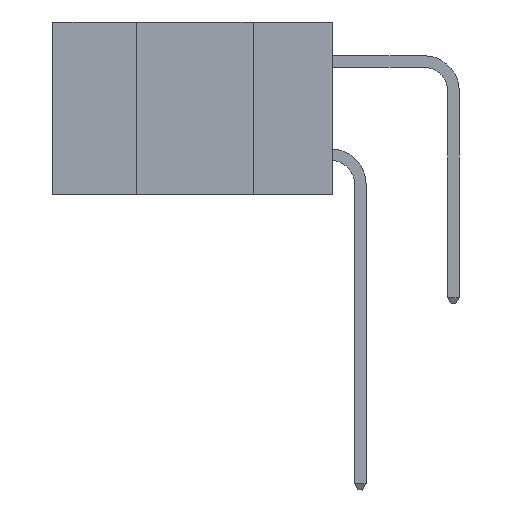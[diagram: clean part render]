
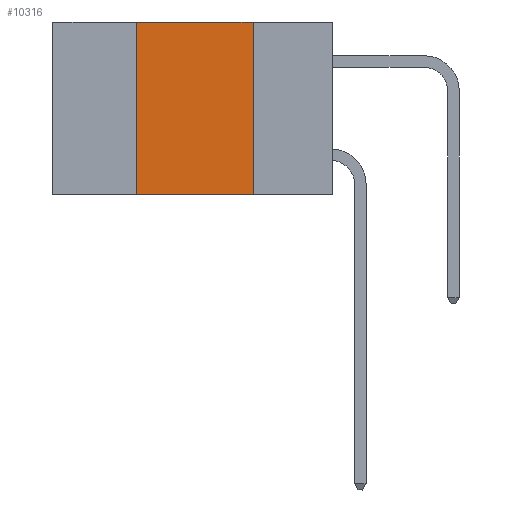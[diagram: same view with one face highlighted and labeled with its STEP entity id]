
A CAD part, left-side view. The second image highlights one B-rep face of the part: STEP entity #10316.
In plain terms, the highlighted planar face has unit normal (-1, 0, 0).
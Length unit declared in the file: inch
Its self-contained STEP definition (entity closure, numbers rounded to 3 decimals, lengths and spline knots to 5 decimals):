
#1430 = CARTESIAN_POINT ( 'NONE',  ( 0., 0.42, 0. ) ) ;
#2302 = LINE ( 'NONE', #6742, #3215 ) ;
#2403 = VECTOR ( 'NONE', #13014, 39.37008 ) ;
#2404 = CARTESIAN_POINT ( 'NONE',  ( 0., 0.6, -0.37 ) ) ;
#2976 = CARTESIAN_POINT ( 'NONE',  ( 0., 0.17, 0. ) ) ;
#3215 = VECTOR ( 'NONE', #18125, 39.37008 ) ;
#3282 = DIRECTION ( 'NONE',  ( 0., 0., 1. ) ) ;
#4327 = LINE ( 'NONE', #2404, #15192 ) ;
#4336 = EDGE_CURVE ( 'NONE', #9946, #16621, #2302, .T. ) ;
#4910 = EDGE_CURVE ( 'NONE', #8265, #6599, #4327, .T. ) ;
#5013 = VECTOR ( 'NONE', #3282, 39.37008 ) ;
#6599 = VERTEX_POINT ( 'NONE', #17805 ) ;
#6646 = DIRECTION ( 'NONE',  ( 1., 0., 0. ) ) ;
#6742 = CARTESIAN_POINT ( 'NONE',  ( 0., 0.6, 0. ) ) ;
#7209 = EDGE_LOOP ( 'NONE', ( #18222, #9034, #10643, #7542 ) ) ;
#7542 = ORIENTED_EDGE ( 'NONE', *, *, #4910, .T. ) ;
#8265 = VERTEX_POINT ( 'NONE', #16292 ) ;
#9034 = ORIENTED_EDGE ( 'NONE', *, *, #4336, .F. ) ;
#9946 = VERTEX_POINT ( 'NONE', #1430 ) ;
#10080 = FACE_OUTER_BOUND ( 'NONE', #7209, .T. ) ;
#10316 = ADVANCED_FACE ( 'NONE', ( #10080 ), #15088, .F. ) ;
#10488 = CARTESIAN_POINT ( 'NONE',  ( 0., 0.42, 0. ) ) ;
#10643 = ORIENTED_EDGE ( 'NONE', *, *, #18179, .F. ) ;
#12333 = CARTESIAN_POINT ( 'NONE',  ( 0., 0.6, 0. ) ) ;
#12358 = AXIS2_PLACEMENT_3D ( 'NONE', #12333, #6646, #16526 ) ;
#12776 = CARTESIAN_POINT ( 'NONE',  ( 0., 0.17, 0. ) ) ;
#13014 = DIRECTION ( 'NONE',  ( 0., 0., -1. ) ) ;
#14239 = LINE ( 'NONE', #2976, #2403 ) ;
#14762 = EDGE_CURVE ( 'NONE', #16621, #6599, #14239, .T. ) ;
#15088 = PLANE ( 'NONE',  #12358 ) ;
#15192 = VECTOR ( 'NONE', #15467, 39.37008 ) ;
#15467 = DIRECTION ( 'NONE',  ( 0., -1., 0. ) ) ;
#16292 = CARTESIAN_POINT ( 'NONE',  ( 0., 0.42, -0.37 ) ) ;
#16338 = LINE ( 'NONE', #10488, #5013 ) ;
#16526 = DIRECTION ( 'NONE',  ( 0., 0., -1. ) ) ;
#16621 = VERTEX_POINT ( 'NONE', #12776 ) ;
#17805 = CARTESIAN_POINT ( 'NONE',  ( 0., 0.17, -0.37 ) ) ;
#18125 = DIRECTION ( 'NONE',  ( 0., -1., 0. ) ) ;
#18179 = EDGE_CURVE ( 'NONE', #8265, #9946, #16338, .T. ) ;
#18222 = ORIENTED_EDGE ( 'NONE', *, *, #14762, .F. ) ;
